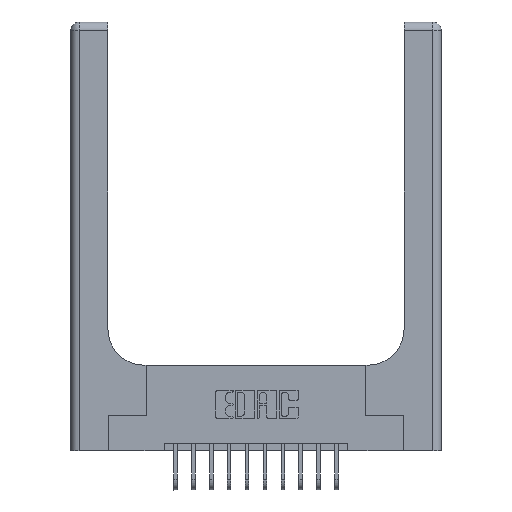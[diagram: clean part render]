
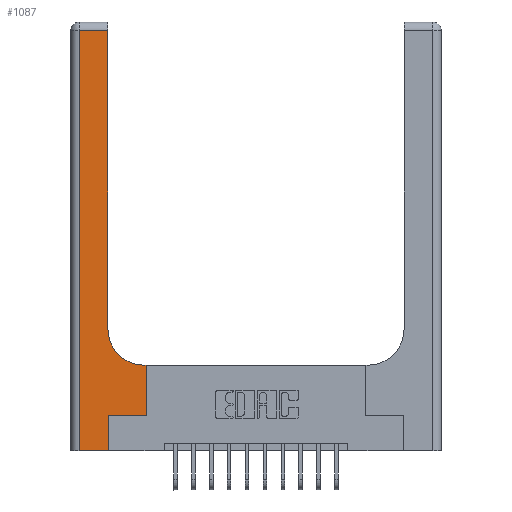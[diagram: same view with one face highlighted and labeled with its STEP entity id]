
A CAD part, top view. The second image highlights one B-rep face of the part: STEP entity #1087.
In plain terms, the highlighted planar face has unit normal (0, 0, 1).
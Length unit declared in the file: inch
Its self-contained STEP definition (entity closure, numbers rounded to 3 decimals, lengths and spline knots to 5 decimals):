
#219 = VECTOR ( 'NONE', #5509, 39.37008 ) ;
#266 = VERTEX_POINT ( 'NONE', #1734 ) ;
#478 = CARTESIAN_POINT ( 'NONE',  ( 0.26, 0.85, 0.37 ) ) ;
#783 = AXIS2_PLACEMENT_3D ( 'NONE', #2999, #8230, #4961 ) ;
#784 = DIRECTION ( 'NONE',  ( -1., 0., 0. ) ) ;
#1087 = ADVANCED_FACE ( 'NONE', ( #15142 ), #15793, .F. ) ;
#1734 = CARTESIAN_POINT ( 'NONE',  ( 0.265, 0., 0.37 ) ) ;
#2325 = ORIENTED_EDGE ( 'NONE', *, *, #13146, .T. ) ;
#2690 = EDGE_CURVE ( 'NONE', #4913, #15060, #14739, .T. ) ;
#2745 = CARTESIAN_POINT ( 'NONE',  ( 0.26, 3., 0.37 ) ) ;
#2999 = CARTESIAN_POINT ( 'NONE',  ( 0., 3., 0.37 ) ) ;
#3109 = LINE ( 'NONE', #3440, #15628 ) ;
#3440 = CARTESIAN_POINT ( 'NONE',  ( 0.265, 0.25, 0.37 ) ) ;
#3454 = VERTEX_POINT ( 'NONE', #4804 ) ;
#3669 = ORIENTED_EDGE ( 'NONE', *, *, #4628, .T. ) ;
#3699 = CARTESIAN_POINT ( 'NONE',  ( 0.51, 0.85, 0.37 ) ) ;
#3781 = ORIENTED_EDGE ( 'NONE', *, *, #5408, .T. ) ;
#3796 = VERTEX_POINT ( 'NONE', #478 ) ;
#4297 = ORIENTED_EDGE ( 'NONE', *, *, #14700, .T. ) ;
#4331 = CARTESIAN_POINT ( 'NONE',  ( 0.26, 2.94, 0.37 ) ) ;
#4466 = VERTEX_POINT ( 'NONE', #7170 ) ;
#4628 = EDGE_CURVE ( 'NONE', #13637, #9877, #12174, .T. ) ;
#4804 = CARTESIAN_POINT ( 'NONE',  ( 0.528, 0.25, 0.37 ) ) ;
#4913 = VERTEX_POINT ( 'NONE', #15287 ) ;
#4920 = DIRECTION ( 'NONE',  ( 1., 0., 0. ) ) ;
#4954 = VECTOR ( 'NONE', #5573, 39.37008 ) ;
#4961 = DIRECTION ( 'NONE',  ( -1., 0., 0. ) ) ;
#5013 = AXIS2_PLACEMENT_3D ( 'NONE', #3699, #12226, #4920 ) ;
#5408 = EDGE_CURVE ( 'NONE', #9877, #4466, #10030, .T. ) ;
#5419 = CIRCLE ( 'NONE', #5013, 0.25 ) ;
#5421 = ORIENTED_EDGE ( 'NONE', *, *, #9569, .T. ) ;
#5509 = DIRECTION ( 'NONE',  ( 0., -1., 0. ) ) ;
#5573 = DIRECTION ( 'NONE',  ( 0., 1., 0. ) ) ;
#6119 = EDGE_LOOP ( 'NONE', ( #2325, #3669, #3781, #4297, #5421, #6872, #10058, #11795, #11899 ) ) ;
#6872 = ORIENTED_EDGE ( 'NONE', *, *, #6968, .T. ) ;
#6968 = EDGE_CURVE ( 'NONE', #9947, #3454, #3109, .T. ) ;
#7170 = CARTESIAN_POINT ( 'NONE',  ( 0.06, 0., 0.37 ) ) ;
#7353 = CARTESIAN_POINT ( 'NONE',  ( 0.265, 0., 0.37 ) ) ;
#7545 = VECTOR ( 'NONE', #8798, 39.37008 ) ;
#8191 = LINE ( 'NONE', #10438, #4954 ) ;
#8230 = DIRECTION ( 'NONE',  ( 0., 0., -1. ) ) ;
#8636 = DIRECTION ( 'NONE',  ( 0., 1., 0. ) ) ;
#8798 = DIRECTION ( 'NONE',  ( 1., 0., 0. ) ) ;
#8896 = LINE ( 'NONE', #2745, #12161 ) ;
#9569 = EDGE_CURVE ( 'NONE', #266, #9947, #12203, .T. ) ;
#9625 = CARTESIAN_POINT ( 'NONE',  ( 0.06, 2.94, 0.37 ) ) ;
#9877 = VERTEX_POINT ( 'NONE', #9625 ) ;
#9947 = VERTEX_POINT ( 'NONE', #12279 ) ;
#10030 = LINE ( 'NONE', #11597, #219 ) ;
#10058 = ORIENTED_EDGE ( 'NONE', *, *, #11729, .T. ) ;
#10438 = CARTESIAN_POINT ( 'NONE',  ( 0.528, 0.25, 0.37 ) ) ;
#10735 = DIRECTION ( 'NONE',  ( 1., 0., 0. ) ) ;
#10765 = VECTOR ( 'NONE', #784, 39.37008 ) ;
#10767 = CARTESIAN_POINT ( 'NONE',  ( 0.51, 0.6, 0.37 ) ) ;
#10789 = LINE ( 'NONE', #14845, #7545 ) ;
#11011 = VECTOR ( 'NONE', #11108, 39.37008 ) ;
#11054 = CARTESIAN_POINT ( 'NONE',  ( 0., 2.94, 0.37 ) ) ;
#11108 = DIRECTION ( 'NONE',  ( -1., 0., 0. ) ) ;
#11597 = CARTESIAN_POINT ( 'NONE',  ( 0.06, 3., 0.37 ) ) ;
#11729 = EDGE_CURVE ( 'NONE', #3454, #4913, #8191, .T. ) ;
#11795 = ORIENTED_EDGE ( 'NONE', *, *, #2690, .T. ) ;
#11899 = ORIENTED_EDGE ( 'NONE', *, *, #13906, .T. ) ;
#12161 = VECTOR ( 'NONE', #12522, 39.37008 ) ;
#12174 = LINE ( 'NONE', #11054, #11011 ) ;
#12203 = LINE ( 'NONE', #7353, #15002 ) ;
#12226 = DIRECTION ( 'NONE',  ( 0., 0., -1. ) ) ;
#12279 = CARTESIAN_POINT ( 'NONE',  ( 0.265, 0.25, 0.37 ) ) ;
#12522 = DIRECTION ( 'NONE',  ( 0., 1., 0. ) ) ;
#13146 = EDGE_CURVE ( 'NONE', #3796, #13637, #8896, .T. ) ;
#13637 = VERTEX_POINT ( 'NONE', #4331 ) ;
#13906 = EDGE_CURVE ( 'NONE', #15060, #3796, #5419, .T. ) ;
#14700 = EDGE_CURVE ( 'NONE', #4466, #266, #10789, .T. ) ;
#14739 = LINE ( 'NONE', #15390, #10765 ) ;
#14845 = CARTESIAN_POINT ( 'NONE',  ( 0., 0., 0.37 ) ) ;
#15002 = VECTOR ( 'NONE', #8636, 39.37008 ) ;
#15060 = VERTEX_POINT ( 'NONE', #10767 ) ;
#15142 = FACE_OUTER_BOUND ( 'NONE', #6119, .T. ) ;
#15287 = CARTESIAN_POINT ( 'NONE',  ( 0.528, 0.6, 0.37 ) ) ;
#15390 = CARTESIAN_POINT ( 'NONE',  ( 0.26, 0.6, 0.37 ) ) ;
#15628 = VECTOR ( 'NONE', #10735, 39.37008 ) ;
#15793 = PLANE ( 'NONE',  #783 ) ;
